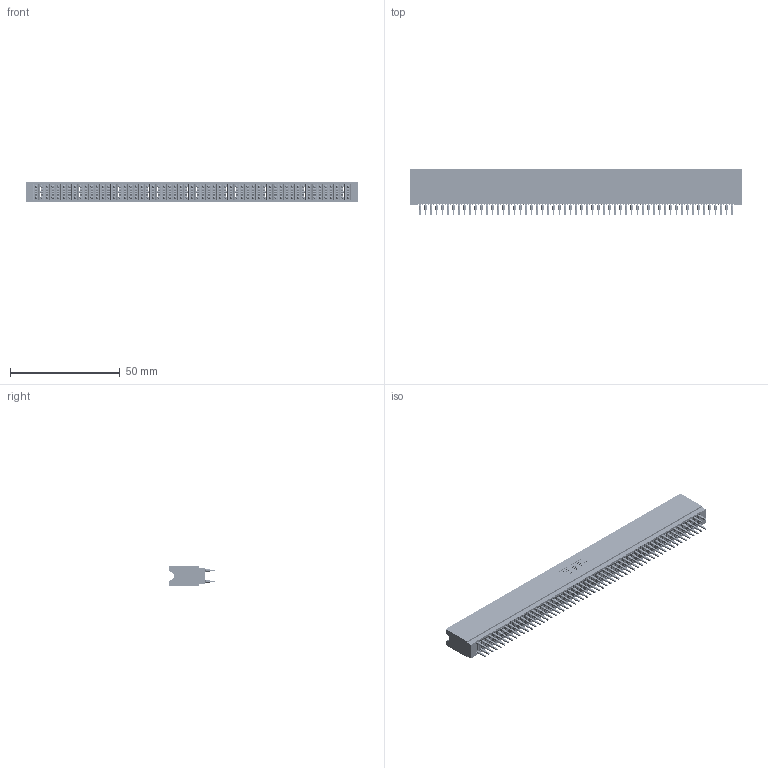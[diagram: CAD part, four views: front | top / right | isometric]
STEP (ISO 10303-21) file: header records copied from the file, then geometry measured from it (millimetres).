
FILE_DESCRIPTION (( 'STEP AP203' ), '1' );
FILE_NAME ('745-114-560-206.STEP', '2026-02-27T00:51:11', ( '' ), ( '' ), 'SwSTEP 2.0', 'SolidWorks 2023', '' );
FILE_SCHEMA (( 'CONFIG_CONTROL_DESIGN' ));
Length unit declared in the file: millimetre
Products named in the file (3): 745-292-001_560; 745 Part_Insulator Option - 06; 745-114-560-206
Assembly tree (115 placements, depth 2):
  745-114-560-206
    745 Part_Insulator Option - 06
    745-292-001_560  x114
Bounding box: 151.38 x 21.22 x 8.89 mm (x, y, z)
Volume: 13941.7 mm3; surface area: 30515.2 mm2
Topology: 115 solids, 115 shells, 11325 faces, 30983 edges, 19666 vertices
Faces by surface type: plane 5870, cylinder 2491, bspline 2280, torus 684
Entity records: 94256 total; most frequent: CARTESIAN_POINT 16848, ORIENTED_EDGE 16314, DIRECTION 14243, EDGE_CURVE 8157, VECTOR 7625, LINE 7625, VERTEX_POINT 5202, AXIS2_PLACEMENT_3D 3309
